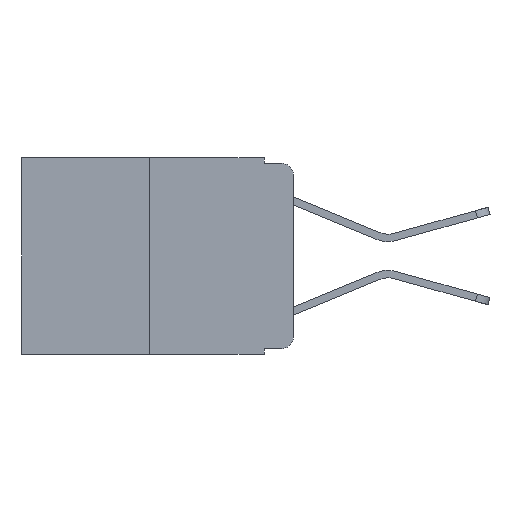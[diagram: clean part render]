
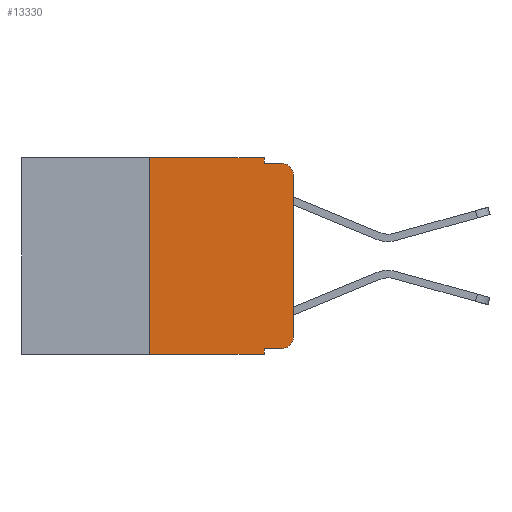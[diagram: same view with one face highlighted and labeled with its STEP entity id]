
A CAD part, left-side view. The second image highlights one B-rep face of the part: STEP entity #13330.
In plain terms, the highlighted planar face has unit normal (-1, 0, 0).
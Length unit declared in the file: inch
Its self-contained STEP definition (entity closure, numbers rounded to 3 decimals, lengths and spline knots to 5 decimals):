
#425 = DIRECTION ( 'NONE',  ( -1., 0., 0. ) ) ;
#834 = CARTESIAN_POINT ( 'NONE',  ( 0., 0.051, -0.333 ) ) ;
#1095 = DIRECTION ( 'NONE',  ( 1., 0., 0. ) ) ;
#1183 = ORIENTED_EDGE ( 'NONE', *, *, #7208, .F. ) ;
#1248 = DIRECTION ( 'NONE',  ( 0., 0., -1. ) ) ;
#1257 = EDGE_CURVE ( 'NONE', #9024, #3416, #5087, .T. ) ;
#1311 = DIRECTION ( 'NONE',  ( 0., -1., 0. ) ) ;
#1345 = CARTESIAN_POINT ( 'NONE',  ( 0., 0.051, 0. ) ) ;
#1493 = CARTESIAN_POINT ( 'NONE',  ( 0., 0.02, -0.333 ) ) ;
#1496 = VECTOR ( 'NONE', #1248, 39.37008 ) ;
#2278 = EDGE_CURVE ( 'NONE', #9185, #19136, #3482, .T. ) ;
#2361 = EDGE_CURVE ( 'NONE', #12564, #5730, #10706, .T. ) ;
#2722 = EDGE_CURVE ( 'NONE', #19136, #12325, #8415, .T. ) ;
#2830 = CARTESIAN_POINT ( 'NONE',  ( 0., 0., 0. ) ) ;
#3272 = CARTESIAN_POINT ( 'NONE',  ( 0., 0.051, -0.01 ) ) ;
#3416 = VERTEX_POINT ( 'NONE', #18722 ) ;
#3482 = LINE ( 'NONE', #2830, #11753 ) ;
#3968 = CARTESIAN_POINT ( 'NONE',  ( 0., 0.25, 0. ) ) ;
#4176 = ORIENTED_EDGE ( 'NONE', *, *, #2722, .T. ) ;
#4772 = DIRECTION ( 'NONE',  ( -1., 0., 0. ) ) ;
#4838 = ORIENTED_EDGE ( 'NONE', *, *, #8019, .F. ) ;
#4932 = DIRECTION ( 'NONE',  ( 0., 0., -1. ) ) ;
#5087 = LINE ( 'NONE', #14141, #10011 ) ;
#5554 = FACE_OUTER_BOUND ( 'NONE', #9828, .T. ) ;
#5630 = DIRECTION ( 'NONE',  ( 0., 0., 1. ) ) ;
#5730 = VERTEX_POINT ( 'NONE', #1345 ) ;
#5787 = DIRECTION ( 'NONE',  ( 0., -1., 0. ) ) ;
#5837 = VECTOR ( 'NONE', #5630, 39.37008 ) ;
#6102 = PLANE ( 'NONE',  #12819 ) ;
#6274 = CIRCLE ( 'NONE', #19447, 0.02 ) ;
#6468 = DIRECTION ( 'NONE',  ( 0., -1., 0. ) ) ;
#7116 = EDGE_CURVE ( 'NONE', #5730, #13372, #14718, .T. ) ;
#7208 = EDGE_CURVE ( 'NONE', #13372, #12325, #21224, .T. ) ;
#7396 = ORIENTED_EDGE ( 'NONE', *, *, #1257, .T. ) ;
#7778 = ORIENTED_EDGE ( 'NONE', *, *, #2361, .F. ) ;
#8019 = EDGE_CURVE ( 'NONE', #9416, #3416, #10817, .T. ) ;
#8264 = CARTESIAN_POINT ( 'NONE',  ( 0., 0.02, -0.01 ) ) ;
#8415 = CIRCLE ( 'NONE', #10599, 0.02 ) ;
#8805 = VECTOR ( 'NONE', #5787, 39.37008 ) ;
#8818 = CARTESIAN_POINT ( 'NONE',  ( 0., 0.473, 0. ) ) ;
#9024 = VERTEX_POINT ( 'NONE', #11506 ) ;
#9185 = VERTEX_POINT ( 'NONE', #18448 ) ;
#9385 = CARTESIAN_POINT ( 'NONE',  ( 0., 0., -0.03 ) ) ;
#9416 = VERTEX_POINT ( 'NONE', #834 ) ;
#9828 = EDGE_LOOP ( 'NONE', ( #10071, #4176, #1183, #19680, #7778, #14554, #7396, #4838, #15679, #12106 ) ) ;
#9833 = EDGE_CURVE ( 'NONE', #9024, #12564, #18867, .T. ) ;
#10011 = VECTOR ( 'NONE', #6468, 39.37008 ) ;
#10071 = ORIENTED_EDGE ( 'NONE', *, *, #2278, .T. ) ;
#10251 = CARTESIAN_POINT ( 'NONE',  ( 0., 0.02, -0.03 ) ) ;
#10459 = CARTESIAN_POINT ( 'NONE',  ( 0., 0.051, 0. ) ) ;
#10461 = CARTESIAN_POINT ( 'NONE',  ( 0., 0.02, -0.313 ) ) ;
#10599 = AXIS2_PLACEMENT_3D ( 'NONE', #10251, #4772, #4932 ) ;
#10706 = LINE ( 'NONE', #8818, #18346 ) ;
#10817 = LINE ( 'NONE', #10459, #18944 ) ;
#11076 = CARTESIAN_POINT ( 'NONE',  ( 0., 0.473, 0. ) ) ;
#11506 = CARTESIAN_POINT ( 'NONE',  ( 0., 0.25, -0.343 ) ) ;
#11753 = VECTOR ( 'NONE', #15988, 39.37008 ) ;
#12106 = ORIENTED_EDGE ( 'NONE', *, *, #14913, .T. ) ;
#12123 = DIRECTION ( 'NONE',  ( 0., 0., -1. ) ) ;
#12325 = VERTEX_POINT ( 'NONE', #8264 ) ;
#12381 = DIRECTION ( 'NONE',  ( 0., -1., 0. ) ) ;
#12564 = VERTEX_POINT ( 'NONE', #13973 ) ;
#12738 = DIRECTION ( 'NONE',  ( 0., 0., -1. ) ) ;
#12819 = AXIS2_PLACEMENT_3D ( 'NONE', #11076, #1095, #12738 ) ;
#13330 = ADVANCED_FACE ( 'NONE', ( #5554 ), #6102, .F. ) ;
#13372 = VERTEX_POINT ( 'NONE', #17683 ) ;
#13973 = CARTESIAN_POINT ( 'NONE',  ( 0., 0.25, 0. ) ) ;
#14141 = CARTESIAN_POINT ( 'NONE',  ( 0., 0.473, -0.343 ) ) ;
#14554 = ORIENTED_EDGE ( 'NONE', *, *, #9833, .F. ) ;
#14718 = LINE ( 'NONE', #20607, #1496 ) ;
#14913 = EDGE_CURVE ( 'NONE', #20664, #9185, #6274, .T. ) ;
#15679 = ORIENTED_EDGE ( 'NONE', *, *, #16627, .T. ) ;
#15988 = DIRECTION ( 'NONE',  ( 0., 0., 1. ) ) ;
#16627 = EDGE_CURVE ( 'NONE', #9416, #20664, #18477, .T. ) ;
#16926 = DIRECTION ( 'NONE',  ( 0., 0., -1. ) ) ;
#17176 = CARTESIAN_POINT ( 'NONE',  ( 0., 0.051, -0.333 ) ) ;
#17683 = CARTESIAN_POINT ( 'NONE',  ( 0., 0.051, -0.01 ) ) ;
#17977 = VECTOR ( 'NONE', #12381, 39.37008 ) ;
#18346 = VECTOR ( 'NONE', #1311, 39.37008 ) ;
#18448 = CARTESIAN_POINT ( 'NONE',  ( 0., 0., -0.313 ) ) ;
#18477 = LINE ( 'NONE', #17176, #17977 ) ;
#18722 = CARTESIAN_POINT ( 'NONE',  ( 0., 0.051, -0.343 ) ) ;
#18867 = LINE ( 'NONE', #3968, #5837 ) ;
#18944 = VECTOR ( 'NONE', #16926, 39.37008 ) ;
#19136 = VERTEX_POINT ( 'NONE', #9385 ) ;
#19447 = AXIS2_PLACEMENT_3D ( 'NONE', #10461, #425, #12123 ) ;
#19680 = ORIENTED_EDGE ( 'NONE', *, *, #7116, .F. ) ;
#20607 = CARTESIAN_POINT ( 'NONE',  ( 0., 0.051, 0. ) ) ;
#20664 = VERTEX_POINT ( 'NONE', #1493 ) ;
#21224 = LINE ( 'NONE', #3272, #8805 ) ;
